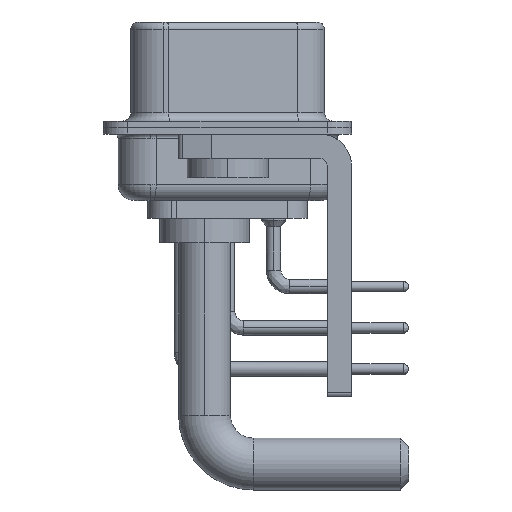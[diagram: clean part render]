
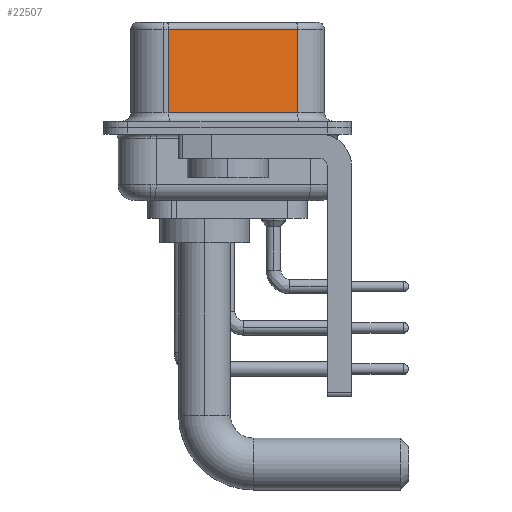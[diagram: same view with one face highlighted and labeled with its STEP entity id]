
A CAD part, left-side view. The second image highlights one B-rep face of the part: STEP entity #22507.
In plain terms, the highlighted planar face has unit normal (-0.985, -0.174, 0).
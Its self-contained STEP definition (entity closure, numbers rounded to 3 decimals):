
#37 = VERTEX_POINT ( 'NONE', #4952 ) ;
#3320 = ORIENTED_EDGE ( 'NONE', *, *, #14033, .F. ) ;
#3572 = LINE ( 'NONE', #25303, #10559 ) ;
#4155 = VECTOR ( 'NONE', #18317, 1000. ) ;
#4783 = VECTOR ( 'NONE', #27465, 1000. ) ;
#4945 = EDGE_CURVE ( 'NONE', #19923, #37, #3572, .T. ) ;
#4952 = CARTESIAN_POINT ( 'NONE',  ( 3.73, 3.628, 6.02 ) ) ;
#5458 = VERTEX_POINT ( 'NONE', #26019 ) ;
#6626 = CARTESIAN_POINT ( 'NONE',  ( 5.132, -4.322, 6.52 ) ) ;
#7085 = DIRECTION ( 'NONE',  ( 0.985, 0.174, 0. ) ) ;
#8247 = CARTESIAN_POINT ( 'NONE',  ( 5.132, -4.322, 0.9 ) ) ;
#10559 = VECTOR ( 'NONE', #24001, 1000. ) ;
#14033 = EDGE_CURVE ( 'NONE', #19923, #5458, #19467, .T. ) ;
#14371 = CARTESIAN_POINT ( 'NONE',  ( 5.132, -4.322, 6.02 ) ) ;
#14389 = AXIS2_PLACEMENT_3D ( 'NONE', #30757, #7085, #17586 ) ;
#17586 = DIRECTION ( 'NONE',  ( -0.174, 0.985, 0. ) ) ;
#18317 = DIRECTION ( 'NONE',  ( 0., 0., -1. ) ) ;
#19028 = CARTESIAN_POINT ( 'NONE',  ( 3.73, 3.628, 6.52 ) ) ;
#19467 = LINE ( 'NONE', #6626, #4783 ) ;
#19923 = VERTEX_POINT ( 'NONE', #14371 ) ;
#19924 = PLANE ( 'NONE',  #14389 ) ;
#21976 = DIRECTION ( 'NONE',  ( 0.174, -0.985, 0. ) ) ;
#22319 = LINE ( 'NONE', #8247, #32226 ) ;
#22507 = ADVANCED_FACE ( 'NONE', ( #31112 ), #19924, .F. ) ;
#24001 = DIRECTION ( 'NONE',  ( -0.174, 0.985, 0. ) ) ;
#24012 = LINE ( 'NONE', #19028, #4155 ) ;
#24475 = ORIENTED_EDGE ( 'NONE', *, *, #34076, .T. ) ;
#25303 = CARTESIAN_POINT ( 'NONE',  ( 5.132, -4.322, 6.02 ) ) ;
#26019 = CARTESIAN_POINT ( 'NONE',  ( 5.132, -4.322, 0.9 ) ) ;
#27341 = ORIENTED_EDGE ( 'NONE', *, *, #28137, .T. ) ;
#27465 = DIRECTION ( 'NONE',  ( 0., 0., -1. ) ) ;
#28137 = EDGE_CURVE ( 'NONE', #33265, #5458, #22319, .T. ) ;
#28442 = EDGE_LOOP ( 'NONE', ( #3320, #31651, #24475, #27341 ) ) ;
#30757 = CARTESIAN_POINT ( 'NONE',  ( 5.132, -4.322, 6.52 ) ) ;
#31112 = FACE_OUTER_BOUND ( 'NONE', #28442, .T. ) ;
#31651 = ORIENTED_EDGE ( 'NONE', *, *, #4945, .T. ) ;
#32226 = VECTOR ( 'NONE', #21976, 1000. ) ;
#33183 = CARTESIAN_POINT ( 'NONE',  ( 3.73, 3.628, 0.9 ) ) ;
#33265 = VERTEX_POINT ( 'NONE', #33183 ) ;
#34076 = EDGE_CURVE ( 'NONE', #37, #33265, #24012, .T. ) ;
